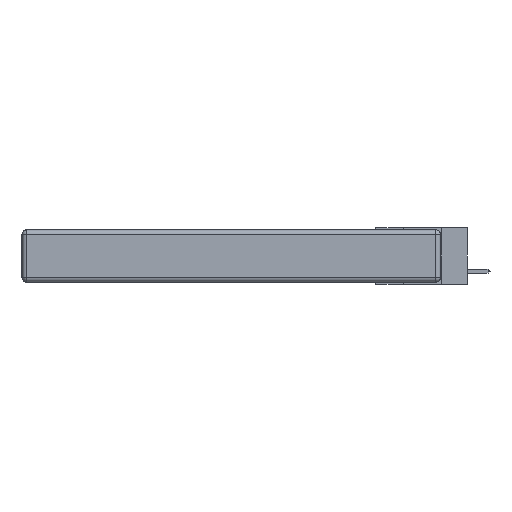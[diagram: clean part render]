
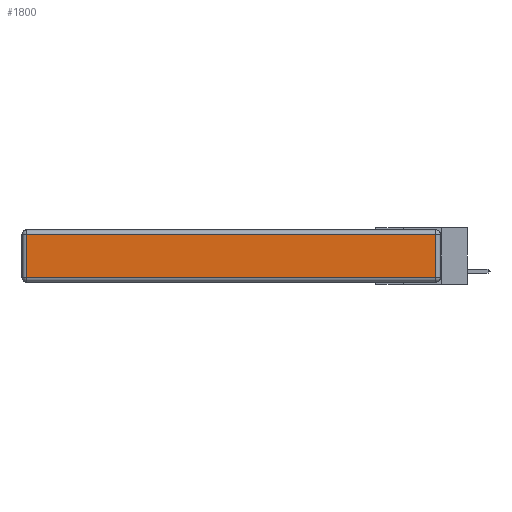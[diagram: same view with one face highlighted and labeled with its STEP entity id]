
A CAD part, left-side view. The second image highlights one B-rep face of the part: STEP entity #1800.
In plain terms, the highlighted planar face has unit normal (-1, 0, 0).
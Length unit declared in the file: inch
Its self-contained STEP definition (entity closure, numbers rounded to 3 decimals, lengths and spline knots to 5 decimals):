
#284 = DIRECTION ( 'NONE',  ( 0., 0., 1. ) ) ;
#445 = EDGE_CURVE ( 'NONE', #3891, #17116, #5206, .T. ) ;
#1278 = VECTOR ( 'NONE', #1395, 39.37008 ) ;
#1395 = DIRECTION ( 'NONE',  ( 0., 1., 0. ) ) ;
#1558 = DIRECTION ( 'NONE',  ( -1., 0., 0. ) ) ;
#1800 = ADVANCED_FACE ( 'NONE', ( #9308 ), #8664, .T. ) ;
#1864 = CARTESIAN_POINT ( 'NONE',  ( 0., 0., -0.313 ) ) ;
#1930 = DIRECTION ( 'NONE',  ( 0., -1., 0. ) ) ;
#1960 = ORIENTED_EDGE ( 'NONE', *, *, #10462, .T. ) ;
#3867 = CARTESIAN_POINT ( 'NONE',  ( 0., 2.72, -0.343 ) ) ;
#3885 = LINE ( 'NONE', #1864, #9771 ) ;
#3891 = VERTEX_POINT ( 'NONE', #9605 ) ;
#4797 = CARTESIAN_POINT ( 'NONE',  ( 0., 0.03, -0.343 ) ) ;
#4928 = ORIENTED_EDGE ( 'NONE', *, *, #10202, .T. ) ;
#5206 = LINE ( 'NONE', #3867, #10677 ) ;
#5896 = VECTOR ( 'NONE', #6178, 39.37008 ) ;
#6178 = DIRECTION ( 'NONE',  ( 0., 0., 1. ) ) ;
#6972 = LINE ( 'NONE', #8134, #1278 ) ;
#8134 = CARTESIAN_POINT ( 'NONE',  ( 0., 2.75, -0.03 ) ) ;
#8424 = VERTEX_POINT ( 'NONE', #11933 ) ;
#8664 = PLANE ( 'NONE',  #13693 ) ;
#8962 = LINE ( 'NONE', #4797, #5896 ) ;
#9060 = ORIENTED_EDGE ( 'NONE', *, *, #11760, .T. ) ;
#9293 = CARTESIAN_POINT ( 'NONE',  ( 0., 2.72, -0.313 ) ) ;
#9308 = FACE_OUTER_BOUND ( 'NONE', #14788, .T. ) ;
#9449 = CARTESIAN_POINT ( 'NONE',  ( 0., 0.03, -0.313 ) ) ;
#9605 = CARTESIAN_POINT ( 'NONE',  ( 0., 2.72, -0.03 ) ) ;
#9771 = VECTOR ( 'NONE', #1930, 39.37008 ) ;
#10202 = EDGE_CURVE ( 'NONE', #8424, #3891, #6972, .T. ) ;
#10462 = EDGE_CURVE ( 'NONE', #12113, #8424, #8962, .T. ) ;
#10677 = VECTOR ( 'NONE', #13643, 39.37008 ) ;
#11760 = EDGE_CURVE ( 'NONE', #17116, #12113, #3885, .T. ) ;
#11933 = CARTESIAN_POINT ( 'NONE',  ( 0., 0.03, -0.03 ) ) ;
#12020 = ORIENTED_EDGE ( 'NONE', *, *, #445, .T. ) ;
#12113 = VERTEX_POINT ( 'NONE', #9449 ) ;
#13643 = DIRECTION ( 'NONE',  ( 0., 0., -1. ) ) ;
#13693 = AXIS2_PLACEMENT_3D ( 'NONE', #15723, #1558, #284 ) ;
#14788 = EDGE_LOOP ( 'NONE', ( #9060, #1960, #4928, #12020 ) ) ;
#15723 = CARTESIAN_POINT ( 'NONE',  ( 0., 0., -0.343 ) ) ;
#17116 = VERTEX_POINT ( 'NONE', #9293 ) ;
